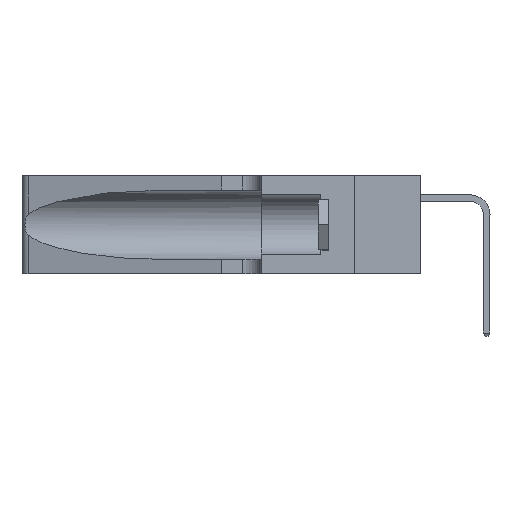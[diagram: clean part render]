
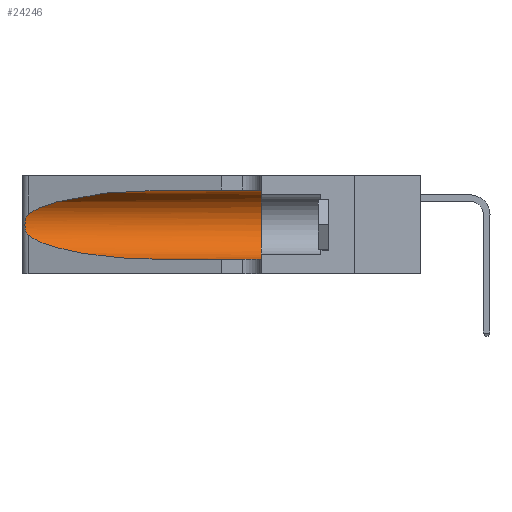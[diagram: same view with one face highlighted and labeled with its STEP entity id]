
A CAD part, left-side view. The second image highlights one B-rep face of the part: STEP entity #24246.
In plain terms, the highlighted cylindrical face has radius 3.308 mm (diameter 6.617 mm), a partial arc.
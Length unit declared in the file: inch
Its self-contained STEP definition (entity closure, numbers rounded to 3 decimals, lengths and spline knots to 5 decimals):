
#1062 = ORIENTED_EDGE ( 'NONE', *, *, #22177, .T. ) ;
#2132 = VERTEX_POINT ( 'NONE', #3228 ) ;
#2545 = CARTESIAN_POINT ( 'NONE',  ( 0.26075, 1.23896, 0.178 ) ) ;
#2669 = EDGE_CURVE ( 'NONE', #27085, #24249, #16286, .T. ) ;
#2862 = ORIENTED_EDGE ( 'NONE', *, *, #2669, .T. ) ;
#3228 = CARTESIAN_POINT ( 'NONE',  ( 0.1305, 0.35, 0.31525 ) ) ;
#3294 = CARTESIAN_POINT ( 'NONE',  ( 0.25487, 1.22718, 0.22369 ) ) ;
#3643 = DIRECTION ( 'NONE',  ( 0., 1., 0. ) ) ;
#3746 = CARTESIAN_POINT ( 'NONE',  ( 0.1305, 1.61858, 0.05475 ) ) ;
#4899 = EDGE_CURVE ( 'NONE', #14698, #27279, #11721, .T. ) ;
#5141 = DIRECTION ( 'NONE',  ( 0., -1., 0. ) ) ;
#5580 = CARTESIAN_POINT ( 'NONE',  ( 0.25856, 1.23593, 0.16098 ) ) ;
#5744 = CIRCLE ( 'NONE', #32643, 0.13025 ) ;
#8088 = ORIENTED_EDGE ( 'NONE', *, *, #23984, .T. ) ;
#8737 = CARTESIAN_POINT ( 'NONE',  ( 0.25639, 1.23186, 0.15144 ) ) ;
#9942 = ORIENTED_EDGE ( 'NONE', *, *, #4899, .T. ) ;
#10750 = DIRECTION ( 'NONE',  ( 0., -1., 0. ) ) ;
#10890 = DIRECTION ( 'NONE',  ( 0., 0., -1. ) ) ;
#11219 = VECTOR ( 'NONE', #21750, 39.37008 ) ;
#11721 = LINE ( 'NONE', #3746, #11219 ) ;
#11729 = EDGE_CURVE ( 'NONE', #33673, #2132, #28528, .T. ) ;
#11867 = ORIENTED_EDGE ( 'NONE', *, *, #22832, .F. ) ;
#11897 = CARTESIAN_POINT ( 'NONE',  ( 0.25487, 1.22718, 0.14631 ) ) ;
#12816 = CARTESIAN_POINT ( 'NONE',  ( 0.25487, 1.22718, 0.14631 ) ) ;
#13976 = CARTESIAN_POINT ( 'NONE',  ( 0.25487, 1.22718, 0.14631 ) ) ;
#13983 = FACE_OUTER_BOUND ( 'NONE', #22900, .T. ) ;
#14698 = VERTEX_POINT ( 'NONE', #19432 ) ;
#14853 = CARTESIAN_POINT ( 'NONE',  ( 0.25487, 1.22718, 0.22369 ) ) ;
#15602 = CARTESIAN_POINT ( 'NONE',  ( 0.1305, 0.72297, 0.31525 ) ) ;
#15857 = CARTESIAN_POINT ( 'NONE',  ( 0.2373, 1.15595, 0.08982 ) ) ;
#16286 = B_SPLINE_CURVE_WITH_KNOTS ( 'NONE', 3,
 ( #14853, #37646, #32003, #34866, #17796, #37772, #20600, #2545, #23544, #5580, #26424, #8737, #29298, #11897 ),
 .UNSPECIFIED., .F., .F.,
 ( 4, 2, 2, 2, 2, 2, 4 ),
 ( 0., 0.00027, 0.00053, 0.00107, 0.0016, 0.00187, 0.00214 ),
 .UNSPECIFIED. ) ;
#17796 = CARTESIAN_POINT ( 'NONE',  ( 0.25854, 1.2359, 0.20912 ) ) ;
#18410 = ORIENTED_EDGE ( 'NONE', *, *, #11729, .F. ) ;
#18731 = CARTESIAN_POINT ( 'NONE',  ( 0.1305, 0.72297, 0.05475 ) ) ;
#19432 = CARTESIAN_POINT ( 'NONE',  ( 0.1305, 0.72297, 0.05475 ) ) ;
#20175 = CARTESIAN_POINT ( 'NONE',  ( 0.1305, 1.61858, 0.31525 ) ) ;
#20600 = CARTESIAN_POINT ( 'NONE',  ( 0.26075, 1.23896, 0.19203 ) ) ;
#21213 = CARTESIAN_POINT ( 'NONE',  ( 0.1305, 0.35, 0.05475 ) ) ;
#21319 = CARTESIAN_POINT ( 'NONE',  ( 0.2373, 1.15595, 0.28018 ) ) ;
#21649 = CARTESIAN_POINT ( 'NONE',  ( 0.1305, 0.35, 0.185 ) ) ;
#21750 = DIRECTION ( 'NONE',  ( 0., -1., 0. ) ) ;
#22177 = EDGE_CURVE ( 'NONE', #33673, #27085, #33289, .T. ) ;
#22832 = EDGE_CURVE ( 'NONE', #2132, #27279, #5744, .T. ) ;
#22900 = EDGE_LOOP ( 'NONE', ( #1062, #2862, #8088, #9942, #11867, #18410 ) ) ;
#23544 = CARTESIAN_POINT ( 'NONE',  ( 0.26017, 1.23833, 0.17102 ) ) ;
#23984 = EDGE_CURVE ( 'NONE', #24249, #14698, #29427, .T. ) ;
#24246 = ADVANCED_FACE ( 'NONE', ( #13983 ), #35992, .F. ) ;
#24249 = VERTEX_POINT ( 'NONE', #13976 ) ;
#24546 = DIRECTION ( 'NONE',  ( 0., 0., 1. ) ) ;
#26424 = CARTESIAN_POINT ( 'NONE',  ( 0.25789, 1.23486, 0.15765 ) ) ;
#27085 = VERTEX_POINT ( 'NONE', #34752 ) ;
#27279 = VERTEX_POINT ( 'NONE', #21213 ) ;
#28093 = VECTOR ( 'NONE', #5141, 39.37008 ) ;
#28391 = CARTESIAN_POINT ( 'NONE',  ( 0.1305, 1.61858, 0.185 ) ) ;
#28528 = LINE ( 'NONE', #20175, #28093 ) ;
#29298 = CARTESIAN_POINT ( 'NONE',  ( 0.25555, 1.22993, 0.14849 ) ) ;
#29427 =( BOUNDED_CURVE ( )  B_SPLINE_CURVE ( 3, ( #12816, #15857, #35845, #18731 ),
 .UNSPECIFIED., .F., .F. ) 
 B_SPLINE_CURVE_WITH_KNOTS ( ( 4, 4 ),
 ( 3.44316, 4.71239 ),
 .UNSPECIFIED. ) 
 CURVE ( )  GEOMETRIC_REPRESENTATION_ITEM ( )  RATIONAL_B_SPLINE_CURVE ( ( 1., 0.87, 0.87, 1. ) ) 
 REPRESENTATION_ITEM ( '' )  );
#31739 = AXIS2_PLACEMENT_3D ( 'NONE', #28391, #10750, #10890 ) ;
#32003 = CARTESIAN_POINT ( 'NONE',  ( 0.25639, 1.23184, 0.21858 ) ) ;
#32230 = CARTESIAN_POINT ( 'NONE',  ( 0.1305, 0.72297, 0.31525 ) ) ;
#32643 = AXIS2_PLACEMENT_3D ( 'NONE', #21649, #3643, #24546 ) ;
#32713 = CARTESIAN_POINT ( 'NONE',  ( 0.18966, 0.96281, 0.31525 ) ) ;
#33289 =( BOUNDED_CURVE ( )  B_SPLINE_CURVE ( 3, ( #15602, #32713, #21319, #3294 ),
 .UNSPECIFIED., .F., .T. ) 
 B_SPLINE_CURVE_WITH_KNOTS ( ( 4, 4 ),
 ( 1.5708, 2.84003 ),
 .UNSPECIFIED. ) 
 CURVE ( )  GEOMETRIC_REPRESENTATION_ITEM ( )  RATIONAL_B_SPLINE_CURVE ( ( 1., 0.87, 0.87, 1. ) ) 
 REPRESENTATION_ITEM ( '' )  );
#33673 = VERTEX_POINT ( 'NONE', #32230 ) ;
#34752 = CARTESIAN_POINT ( 'NONE',  ( 0.25487, 1.22718, 0.22369 ) ) ;
#34866 = CARTESIAN_POINT ( 'NONE',  ( 0.25787, 1.23484, 0.2124 ) ) ;
#35845 = CARTESIAN_POINT ( 'NONE',  ( 0.18966, 0.96281, 0.05475 ) ) ;
#35992 = CYLINDRICAL_SURFACE ( 'NONE', #31739, 0.13025 ) ;
#37646 = CARTESIAN_POINT ( 'NONE',  ( 0.25555, 1.22994, 0.2215 ) ) ;
#37772 = CARTESIAN_POINT ( 'NONE',  ( 0.26018, 1.23835, 0.19895 ) ) ;
